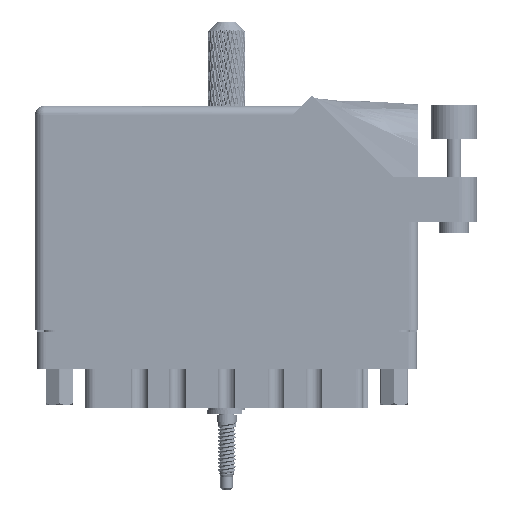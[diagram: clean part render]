
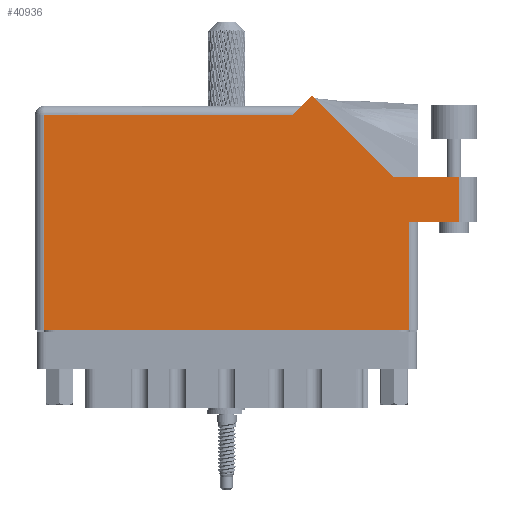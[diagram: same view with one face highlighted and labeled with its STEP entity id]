
A CAD part, front view. The second image highlights one B-rep face of the part: STEP entity #40936.
In plain terms, the highlighted face is planar.
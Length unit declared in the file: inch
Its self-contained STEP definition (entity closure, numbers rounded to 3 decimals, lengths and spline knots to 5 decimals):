
#2205 = DIRECTION ( 'NONE',  ( -1., 0., 0. ) ) ;
#3348 = DIRECTION ( 'NONE',  ( -1., 0., 0. ) ) ;
#3925 = DIRECTION ( 'NONE',  ( -0.707, 0.707, 0. ) ) ;
#5440 = EDGE_CURVE ( 'NONE', #26138, #87900, #13201, .T. ) ;
#9792 = EDGE_CURVE ( 'NONE', #110115, #27804, #110094, .T. ) ;
#10118 = VECTOR ( 'NONE', #118902, 39.37008 ) ;
#13201 = LINE ( 'NONE', #90475, #88966 ) ;
#13732 = VECTOR ( 'NONE', #24365, 39.37008 ) ;
#14364 = CARTESIAN_POINT ( 'NONE',  ( 2.612, 0.737, 0. ) ) ;
#22074 = CARTESIAN_POINT ( 'NONE',  ( 2.887, 1.044, 0. ) ) ;
#22671 = LINE ( 'NONE', #101495, #31831 ) ;
#24365 = DIRECTION ( 'NONE',  ( -0.707, -0.707, 0. ) ) ;
#26138 = VERTEX_POINT ( 'NONE', #37771 ) ;
#27068 = ORIENTED_EDGE ( 'NONE', *, *, #101604, .T. ) ;
#27691 = LINE ( 'NONE', #14364, #66339 ) ;
#27783 = VECTOR ( 'NONE', #57111, 39.37008 ) ;
#27804 = VERTEX_POINT ( 'NONE', #105048 ) ;
#28703 = ORIENTED_EDGE ( 'NONE', *, *, #110296, .T. ) ;
#30172 = CARTESIAN_POINT ( 'NONE',  ( 0., 0., 0. ) ) ;
#31831 = VECTOR ( 'NONE', #2205, 39.37008 ) ;
#33012 = DIRECTION ( 'NONE',  ( 0., 0., -1. ) ) ;
#35068 = EDGE_CURVE ( 'NONE', #56584, #26138, #22671, .T. ) ;
#35257 = LINE ( 'NONE', #54620, #13732 ) ;
#36913 = ORIENTED_EDGE ( 'NONE', *, *, #66027, .T. ) ;
#37771 = CARTESIAN_POINT ( 'NONE',  ( 0.062, 1.468, 0. ) ) ;
#39883 = VERTEX_POINT ( 'NONE', #61146 ) ;
#40936 = ADVANCED_FACE ( 'NONE', ( #45361 ), #42530, .F. ) ;
#42530 = PLANE ( 'NONE',  #86356 ) ;
#45361 = FACE_OUTER_BOUND ( 'NONE', #59903, .T. ) ;
#45703 = DIRECTION ( 'NONE',  ( 0., 1., 0. ) ) ;
#49224 = ORIENTED_EDGE ( 'NONE', *, *, #106529, .T. ) ;
#51843 = CARTESIAN_POINT ( 'NONE',  ( 0.062, 0., 0. ) ) ;
#52309 = VECTOR ( 'NONE', #45703, 39.37008 ) ;
#52439 = CARTESIAN_POINT ( 'NONE',  ( 0., 1.53, 0. ) ) ;
#52461 = LINE ( 'NONE', #125916, #27783 ) ;
#54620 = CARTESIAN_POINT ( 'NONE',  ( 1.819, 1.53, 0. ) ) ;
#54917 = EDGE_CURVE ( 'NONE', #95844, #89956, #52461, .T. ) ;
#56584 = VERTEX_POINT ( 'NONE', #126077 ) ;
#57111 = DIRECTION ( 'NONE',  ( 0., 1., 0. ) ) ;
#58764 = LINE ( 'NONE', #114038, #78896 ) ;
#59903 = EDGE_LOOP ( 'NONE', ( #120461, #28703, #73064, #27068, #36913, #107927, #123609, #49224, #87656 ) ) ;
#61146 = CARTESIAN_POINT ( 'NONE',  ( 1.88971, 1.60071, 0. ) ) ;
#61598 = LINE ( 'NONE', #84219, #52309 ) ;
#66027 = EDGE_CURVE ( 'NONE', #39883, #56584, #35257, .T. ) ;
#66339 = VECTOR ( 'NONE', #83474, 39.37008 ) ;
#69540 = CARTESIAN_POINT ( 'NONE',  ( 3.012, 1.044, 0. ) ) ;
#70537 = DIRECTION ( 'NONE',  ( 0., -1., 0. ) ) ;
#73064 = ORIENTED_EDGE ( 'NONE', *, *, #9792, .T. ) ;
#78896 = VECTOR ( 'NONE', #3925, 39.37008 ) ;
#83474 = DIRECTION ( 'NONE',  ( 1., 0., 0. ) ) ;
#84219 = CARTESIAN_POINT ( 'NONE',  ( 2.887, 1.044, 0. ) ) ;
#86356 = AXIS2_PLACEMENT_3D ( 'NONE', #52439, #33012, #3348 ) ;
#87656 = ORIENTED_EDGE ( 'NONE', *, *, #54917, .T. ) ;
#87900 = VERTEX_POINT ( 'NONE', #51843 ) ;
#88966 = VECTOR ( 'NONE', #70537, 39.37008 ) ;
#89058 = DIRECTION ( 'NONE',  ( -1., 0., 0. ) ) ;
#89956 = VERTEX_POINT ( 'NONE', #96476 ) ;
#90475 = CARTESIAN_POINT ( 'NONE',  ( 0.062, 0., 0. ) ) ;
#95844 = VERTEX_POINT ( 'NONE', #104500 ) ;
#96476 = CARTESIAN_POINT ( 'NONE',  ( 2.55, 0.737, 0. ) ) ;
#96649 = LINE ( 'NONE', #30172, #10118 ) ;
#99265 = VECTOR ( 'NONE', #89058, 39.37008 ) ;
#101495 = CARTESIAN_POINT ( 'NONE',  ( 0., 1.468, 0. ) ) ;
#101604 = EDGE_CURVE ( 'NONE', #27804, #39883, #58764, .T. ) ;
#104210 = CARTESIAN_POINT ( 'NONE',  ( 2.887, 0.737, 0. ) ) ;
#104500 = CARTESIAN_POINT ( 'NONE',  ( 2.55, 0., 0. ) ) ;
#105048 = CARTESIAN_POINT ( 'NONE',  ( 2.44642, 1.044, 0. ) ) ;
#106529 = EDGE_CURVE ( 'NONE', #87900, #95844, #96649, .T. ) ;
#107927 = ORIENTED_EDGE ( 'NONE', *, *, #35068, .T. ) ;
#108974 = VERTEX_POINT ( 'NONE', #104210 ) ;
#110094 = LINE ( 'NONE', #69540, #99265 ) ;
#110115 = VERTEX_POINT ( 'NONE', #22074 ) ;
#110296 = EDGE_CURVE ( 'NONE', #108974, #110115, #61598, .T. ) ;
#114038 = CARTESIAN_POINT ( 'NONE',  ( 2.44642, 1.044, 0. ) ) ;
#118902 = DIRECTION ( 'NONE',  ( 1., 0., 0. ) ) ;
#119076 = EDGE_CURVE ( 'NONE', #89956, #108974, #27691, .T. ) ;
#120461 = ORIENTED_EDGE ( 'NONE', *, *, #119076, .T. ) ;
#123609 = ORIENTED_EDGE ( 'NONE', *, *, #5440, .T. ) ;
#125916 = CARTESIAN_POINT ( 'NONE',  ( 2.55, 0.737, 0. ) ) ;
#126077 = CARTESIAN_POINT ( 'NONE',  ( 1.757, 1.468, 0. ) ) ;
